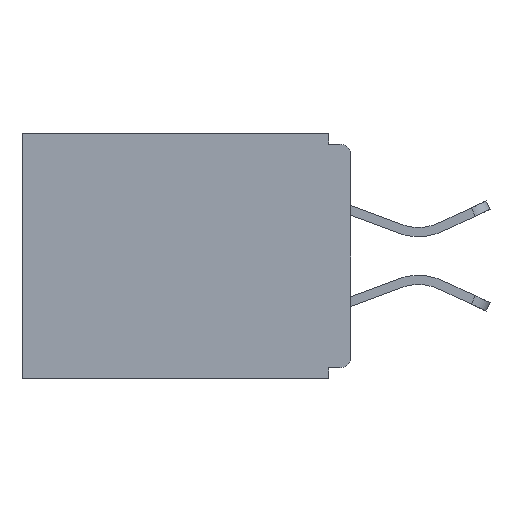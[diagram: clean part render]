
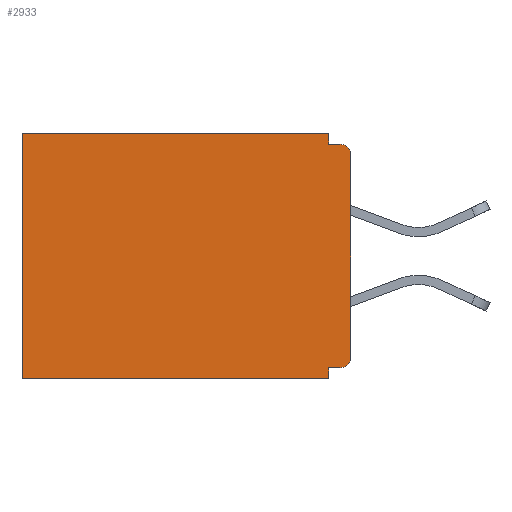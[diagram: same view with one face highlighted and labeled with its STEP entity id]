
A CAD part, left-side view. The second image highlights one B-rep face of the part: STEP entity #2933.
In plain terms, the highlighted planar face has unit normal (-1, 0, 0).
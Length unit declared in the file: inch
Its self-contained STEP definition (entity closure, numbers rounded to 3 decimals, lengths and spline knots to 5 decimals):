
#241 = CARTESIAN_POINT ( 'NONE',  ( 0.298, 0.015, -0.328 ) ) ;
#351 = VERTEX_POINT ( 'NONE', #3296 ) ;
#863 = DIRECTION ( 'NONE',  ( 0., 0., -1. ) ) ;
#904 = EDGE_CURVE ( 'NONE', #1494, #14910, #9796, .T. ) ;
#989 = ORIENTED_EDGE ( 'NONE', *, *, #2420, .F. ) ;
#1270 = VERTEX_POINT ( 'NONE', #241 ) ;
#1307 = LINE ( 'NONE', #4954, #13585 ) ;
#1326 = CARTESIAN_POINT ( 'NONE',  ( 0.298, 0., -0.328 ) ) ;
#1494 = VERTEX_POINT ( 'NONE', #14253 ) ;
#1675 = CARTESIAN_POINT ( 'NONE',  ( 0.298, 0.46, 0. ) ) ;
#2133 = DIRECTION ( 'NONE',  ( -1., 0., 0. ) ) ;
#2292 = VECTOR ( 'NONE', #17980, 39.37008 ) ;
#2314 = ORIENTED_EDGE ( 'NONE', *, *, #11180, .T. ) ;
#2420 = EDGE_CURVE ( 'NONE', #16423, #14910, #1307, .T. ) ;
#2438 = EDGE_LOOP ( 'NONE', ( #11872, #989, #4600, #4559, #2314, #7429, #9718, #13957, #12781, #14858 ) ) ;
#2650 = LINE ( 'NONE', #18466, #10206 ) ;
#2778 = CARTESIAN_POINT ( 'NONE',  ( 0.298, 0.031, -0.343 ) ) ;
#2933 = ADVANCED_FACE ( 'NONE', ( #14665 ), #16405, .F. ) ;
#3296 = CARTESIAN_POINT ( 'NONE',  ( 0.298, 0.46, -0.343 ) ) ;
#3436 = CARTESIAN_POINT ( 'NONE',  ( 0.298, 0.015, -0.03 ) ) ;
#3519 = CARTESIAN_POINT ( 'NONE',  ( 0.298, 0.031, 0. ) ) ;
#4344 = EDGE_CURVE ( 'NONE', #1494, #15294, #6073, .T. ) ;
#4559 = ORIENTED_EDGE ( 'NONE', *, *, #6487, .T. ) ;
#4600 = ORIENTED_EDGE ( 'NONE', *, *, #17045, .F. ) ;
#4954 = CARTESIAN_POINT ( 'NONE',  ( 0.298, 0., -0.015 ) ) ;
#5780 = EDGE_CURVE ( 'NONE', #1270, #14098, #12278, .T. ) ;
#6067 = LINE ( 'NONE', #11892, #13225 ) ;
#6073 = LINE ( 'NONE', #16489, #2292 ) ;
#6111 = DIRECTION ( 'NONE',  ( 0., 0., -1. ) ) ;
#6487 = EDGE_CURVE ( 'NONE', #15024, #13260, #7798, .T. ) ;
#6641 = DIRECTION ( 'NONE',  ( 0., 1., 0. ) ) ;
#6774 = CARTESIAN_POINT ( 'NONE',  ( 0.298, 0.031, -0.343 ) ) ;
#6930 = LINE ( 'NONE', #6774, #15878 ) ;
#7429 = ORIENTED_EDGE ( 'NONE', *, *, #15664, .F. ) ;
#7780 = EDGE_CURVE ( 'NONE', #1270, #15294, #9524, .T. ) ;
#7798 = LINE ( 'NONE', #15260, #13814 ) ;
#8173 = DIRECTION ( 'NONE',  ( 0., -1., 0. ) ) ;
#8290 = CARTESIAN_POINT ( 'NONE',  ( 0.298, 0.031, -0.015 ) ) ;
#8492 = DIRECTION ( 'NONE',  ( 0., 1., 0. ) ) ;
#9524 = CIRCLE ( 'NONE', #18129, 0.015 ) ;
#9718 = ORIENTED_EDGE ( 'NONE', *, *, #17982, .F. ) ;
#9796 = CIRCLE ( 'NONE', #17427, 0.015 ) ;
#9941 = DIRECTION ( 'NONE',  ( 0., 0., -1. ) ) ;
#10206 = VECTOR ( 'NONE', #18343, 39.37008 ) ;
#10284 = DIRECTION ( 'NONE',  ( 0., 1., 0. ) ) ;
#11180 = EDGE_CURVE ( 'NONE', #13260, #351, #2650, .T. ) ;
#11425 = CARTESIAN_POINT ( 'NONE',  ( 0.298, 0.015, -0.313 ) ) ;
#11481 = VERTEX_POINT ( 'NONE', #11710 ) ;
#11710 = CARTESIAN_POINT ( 'NONE',  ( 0.298, 0.031, -0.343 ) ) ;
#11872 = ORIENTED_EDGE ( 'NONE', *, *, #904, .T. ) ;
#11892 = CARTESIAN_POINT ( 'NONE',  ( 0.298, 0., -0.343 ) ) ;
#12151 = DIRECTION ( 'NONE',  ( 1., 0., 0. ) ) ;
#12278 = LINE ( 'NONE', #1326, #15431 ) ;
#12781 = ORIENTED_EDGE ( 'NONE', *, *, #7780, .T. ) ;
#12787 = DIRECTION ( 'NONE',  ( -1., 0., 0. ) ) ;
#13073 = DIRECTION ( 'NONE',  ( 0., 0., -1. ) ) ;
#13225 = VECTOR ( 'NONE', #10284, 39.37008 ) ;
#13260 = VERTEX_POINT ( 'NONE', #1675 ) ;
#13585 = VECTOR ( 'NONE', #8173, 39.37008 ) ;
#13588 = DIRECTION ( 'NONE',  ( 0., 0., -1. ) ) ;
#13814 = VECTOR ( 'NONE', #6641, 39.37008 ) ;
#13957 = ORIENTED_EDGE ( 'NONE', *, *, #5780, .F. ) ;
#14098 = VERTEX_POINT ( 'NONE', #14548 ) ;
#14253 = CARTESIAN_POINT ( 'NONE',  ( 0.298, 0., -0.03 ) ) ;
#14548 = CARTESIAN_POINT ( 'NONE',  ( 0.298, 0.031, -0.328 ) ) ;
#14665 = FACE_OUTER_BOUND ( 'NONE', #2438, .T. ) ;
#14701 = LINE ( 'NONE', #2778, #17170 ) ;
#14858 = ORIENTED_EDGE ( 'NONE', *, *, #4344, .F. ) ;
#14910 = VERTEX_POINT ( 'NONE', #17498 ) ;
#15024 = VERTEX_POINT ( 'NONE', #3519 ) ;
#15260 = CARTESIAN_POINT ( 'NONE',  ( 0.298, 0., 0. ) ) ;
#15294 = VERTEX_POINT ( 'NONE', #17034 ) ;
#15431 = VECTOR ( 'NONE', #8492, 39.37008 ) ;
#15664 = EDGE_CURVE ( 'NONE', #11481, #351, #6067, .T. ) ;
#15878 = VECTOR ( 'NONE', #863, 39.37008 ) ;
#16405 = PLANE ( 'NONE',  #17819 ) ;
#16423 = VERTEX_POINT ( 'NONE', #8290 ) ;
#16472 = CARTESIAN_POINT ( 'NONE',  ( 0.298, 0., 0. ) ) ;
#16489 = CARTESIAN_POINT ( 'NONE',  ( 0.298, 0., 0. ) ) ;
#17034 = CARTESIAN_POINT ( 'NONE',  ( 0.298, 0., -0.313 ) ) ;
#17045 = EDGE_CURVE ( 'NONE', #15024, #16423, #6930, .T. ) ;
#17170 = VECTOR ( 'NONE', #13073, 39.37008 ) ;
#17427 = AXIS2_PLACEMENT_3D ( 'NONE', #3436, #2133, #6111 ) ;
#17498 = CARTESIAN_POINT ( 'NONE',  ( 0.298, 0.015, -0.015 ) ) ;
#17819 = AXIS2_PLACEMENT_3D ( 'NONE', #16472, #12151, #13588 ) ;
#17980 = DIRECTION ( 'NONE',  ( 0., 0., -1. ) ) ;
#17982 = EDGE_CURVE ( 'NONE', #14098, #11481, #14701, .T. ) ;
#18129 = AXIS2_PLACEMENT_3D ( 'NONE', #11425, #12787, #9941 ) ;
#18343 = DIRECTION ( 'NONE',  ( 0., 0., -1. ) ) ;
#18466 = CARTESIAN_POINT ( 'NONE',  ( 0.298, 0.46, 0. ) ) ;
